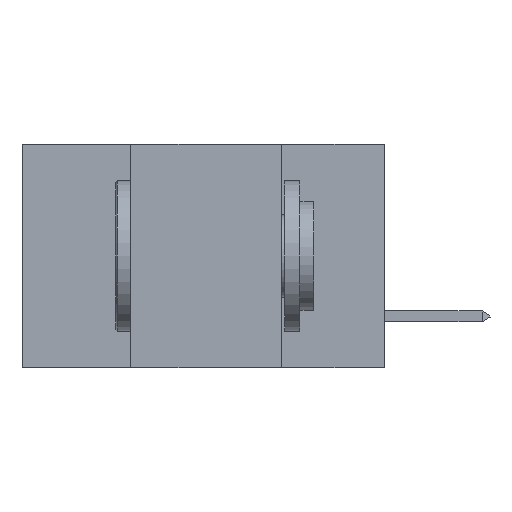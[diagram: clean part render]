
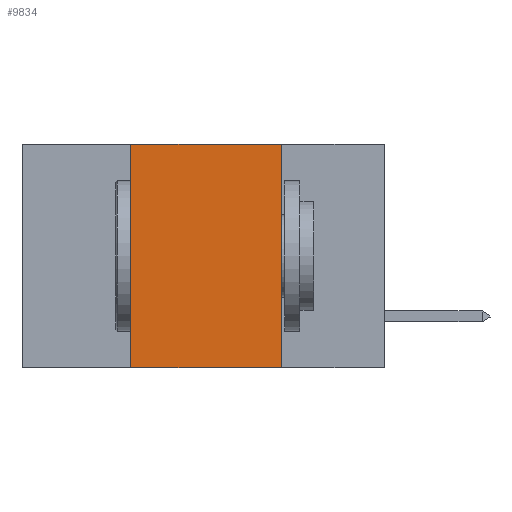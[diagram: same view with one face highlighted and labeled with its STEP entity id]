
A CAD part, left-side view. The second image highlights one B-rep face of the part: STEP entity #9834.
In plain terms, the highlighted planar face has unit normal (-1, 0, 0).
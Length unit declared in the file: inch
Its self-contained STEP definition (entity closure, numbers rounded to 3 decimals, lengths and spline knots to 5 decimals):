
#387 = EDGE_LOOP ( 'NONE', ( #3055, #3098, #3536, #3706 ) ) ;
#555 = CARTESIAN_POINT ( 'NONE',  ( 0., 0.17, 0. ) ) ;
#748 = DIRECTION ( 'NONE',  ( 0., 0., -1. ) ) ;
#1023 = CARTESIAN_POINT ( 'NONE',  ( 0., 0.42, 0. ) ) ;
#1868 = VECTOR ( 'NONE', #748, 39.37008 ) ;
#2090 = CARTESIAN_POINT ( 'NONE',  ( 0., 0.6, 0. ) ) ;
#2346 = CARTESIAN_POINT ( 'NONE',  ( 0., 0.6, 0. ) ) ;
#2353 = EDGE_CURVE ( 'NONE', #6883, #6638, #12314, .T. ) ;
#2435 = CARTESIAN_POINT ( 'NONE',  ( 0., 0.6, -0.37 ) ) ;
#2912 = VECTOR ( 'NONE', #8280, 39.37008 ) ;
#3055 = ORIENTED_EDGE ( 'NONE', *, *, #2353, .F. ) ;
#3098 = ORIENTED_EDGE ( 'NONE', *, *, #8076, .F. ) ;
#3145 = DIRECTION ( 'NONE',  ( 0., 0., -1. ) ) ;
#3536 = ORIENTED_EDGE ( 'NONE', *, *, #12593, .F. ) ;
#3706 = ORIENTED_EDGE ( 'NONE', *, *, #8120, .T. ) ;
#5048 = PLANE ( 'NONE',  #6112 ) ;
#5311 = CARTESIAN_POINT ( 'NONE',  ( 0., 0.42, 0. ) ) ;
#5479 = LINE ( 'NONE', #2346, #10713 ) ;
#5529 = LINE ( 'NONE', #5311, #2912 ) ;
#5617 = VERTEX_POINT ( 'NONE', #1023 ) ;
#6112 = AXIS2_PLACEMENT_3D ( 'NONE', #2090, #9011, #3145 ) ;
#6638 = VERTEX_POINT ( 'NONE', #9058 ) ;
#6883 = VERTEX_POINT ( 'NONE', #555 ) ;
#7503 = LINE ( 'NONE', #2435, #9740 ) ;
#8076 = EDGE_CURVE ( 'NONE', #5617, #6883, #5479, .T. ) ;
#8120 = EDGE_CURVE ( 'NONE', #9781, #6638, #7503, .T. ) ;
#8280 = DIRECTION ( 'NONE',  ( 0., 0., 1. ) ) ;
#9011 = DIRECTION ( 'NONE',  ( 1., 0., 0. ) ) ;
#9058 = CARTESIAN_POINT ( 'NONE',  ( 0., 0.17, -0.37 ) ) ;
#9236 = DIRECTION ( 'NONE',  ( 0., -1., 0. ) ) ;
#9740 = VECTOR ( 'NONE', #12208, 39.37008 ) ;
#9781 = VERTEX_POINT ( 'NONE', #9843 ) ;
#9834 = ADVANCED_FACE ( 'NONE', ( #12164 ), #5048, .F. ) ;
#9843 = CARTESIAN_POINT ( 'NONE',  ( 0., 0.42, -0.37 ) ) ;
#10713 = VECTOR ( 'NONE', #9236, 39.37008 ) ;
#11709 = CARTESIAN_POINT ( 'NONE',  ( 0., 0.17, 0. ) ) ;
#12164 = FACE_OUTER_BOUND ( 'NONE', #387, .T. ) ;
#12208 = DIRECTION ( 'NONE',  ( 0., -1., 0. ) ) ;
#12314 = LINE ( 'NONE', #11709, #1868 ) ;
#12593 = EDGE_CURVE ( 'NONE', #9781, #5617, #5529, .T. ) ;
